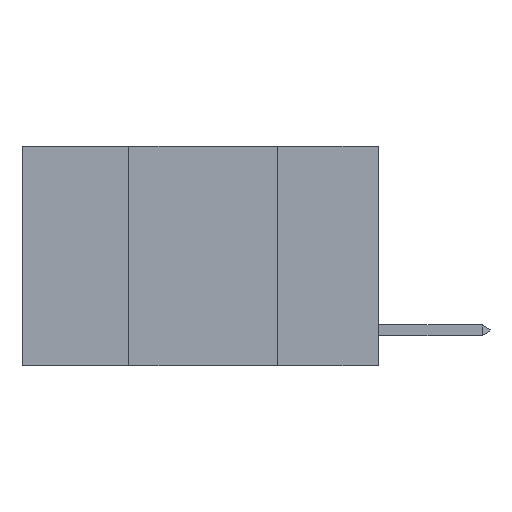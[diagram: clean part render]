
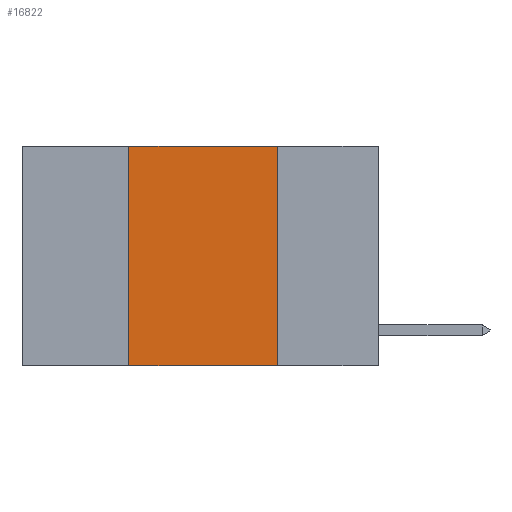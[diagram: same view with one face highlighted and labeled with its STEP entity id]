
A CAD part, left-side view. The second image highlights one B-rep face of the part: STEP entity #16822.
In plain terms, the highlighted planar face has unit normal (-1, 0, 0).
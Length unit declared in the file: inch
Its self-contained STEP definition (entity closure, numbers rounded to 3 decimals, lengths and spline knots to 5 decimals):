
#279 = CARTESIAN_POINT ( 'NONE',  ( 0., 0.17, 0. ) ) ;
#407 = LINE ( 'NONE', #2321, #10608 ) ;
#580 = ORIENTED_EDGE ( 'NONE', *, *, #6484, .F. ) ;
#828 = DIRECTION ( 'NONE',  ( 0., 0., 1. ) ) ;
#1972 = PLANE ( 'NONE',  #5108 ) ;
#2321 = CARTESIAN_POINT ( 'NONE',  ( 0., 0.42, 0. ) ) ;
#2417 = ORIENTED_EDGE ( 'NONE', *, *, #16368, .F. ) ;
#2605 = CARTESIAN_POINT ( 'NONE',  ( 0., 0.17, -0.37 ) ) ;
#3061 = CARTESIAN_POINT ( 'NONE',  ( 0., 0.42, -0.37 ) ) ;
#3365 = DIRECTION ( 'NONE',  ( 0., 0., -1. ) ) ;
#3482 = ORIENTED_EDGE ( 'NONE', *, *, #8543, .T. ) ;
#4068 = VECTOR ( 'NONE', #16871, 39.37008 ) ;
#4709 = LINE ( 'NONE', #14348, #4068 ) ;
#4743 = VERTEX_POINT ( 'NONE', #279 ) ;
#5108 = AXIS2_PLACEMENT_3D ( 'NONE', #7256, #14220, #3365 ) ;
#6484 = EDGE_CURVE ( 'NONE', #4743, #15832, #4709, .T. ) ;
#6671 = FACE_OUTER_BOUND ( 'NONE', #6968, .T. ) ;
#6968 = EDGE_LOOP ( 'NONE', ( #580, #2417, #7724, #3482 ) ) ;
#7256 = CARTESIAN_POINT ( 'NONE',  ( 0., 0.6, 0. ) ) ;
#7581 = DIRECTION ( 'NONE',  ( 0., -1., 0. ) ) ;
#7724 = ORIENTED_EDGE ( 'NONE', *, *, #15007, .F. ) ;
#8406 = VERTEX_POINT ( 'NONE', #10813 ) ;
#8425 = LINE ( 'NONE', #11288, #8655 ) ;
#8543 = EDGE_CURVE ( 'NONE', #11225, #15832, #8425, .T. ) ;
#8655 = VECTOR ( 'NONE', #16544, 39.37008 ) ;
#10285 = CARTESIAN_POINT ( 'NONE',  ( 0., 0.6, 0. ) ) ;
#10608 = VECTOR ( 'NONE', #828, 39.37008 ) ;
#10813 = CARTESIAN_POINT ( 'NONE',  ( 0., 0.42, 0. ) ) ;
#11225 = VERTEX_POINT ( 'NONE', #3061 ) ;
#11288 = CARTESIAN_POINT ( 'NONE',  ( 0., 0.6, -0.37 ) ) ;
#12025 = VECTOR ( 'NONE', #7581, 39.37008 ) ;
#14220 = DIRECTION ( 'NONE',  ( 1., 0., 0. ) ) ;
#14348 = CARTESIAN_POINT ( 'NONE',  ( 0., 0.17, 0. ) ) ;
#15007 = EDGE_CURVE ( 'NONE', #11225, #8406, #407, .T. ) ;
#15832 = VERTEX_POINT ( 'NONE', #2605 ) ;
#16059 = LINE ( 'NONE', #10285, #12025 ) ;
#16368 = EDGE_CURVE ( 'NONE', #8406, #4743, #16059, .T. ) ;
#16544 = DIRECTION ( 'NONE',  ( 0., -1., 0. ) ) ;
#16822 = ADVANCED_FACE ( 'NONE', ( #6671 ), #1972, .F. ) ;
#16871 = DIRECTION ( 'NONE',  ( 0., 0., -1. ) ) ;
